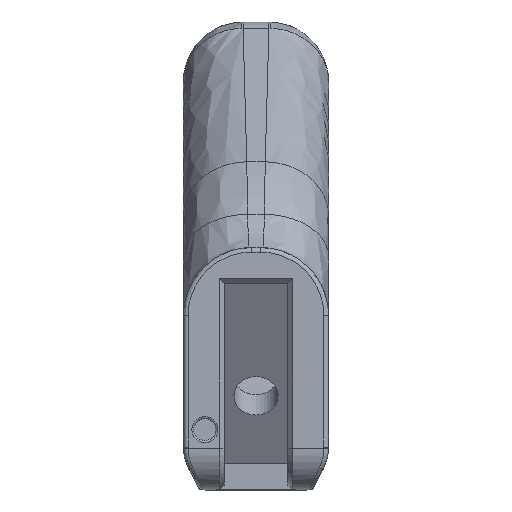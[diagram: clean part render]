
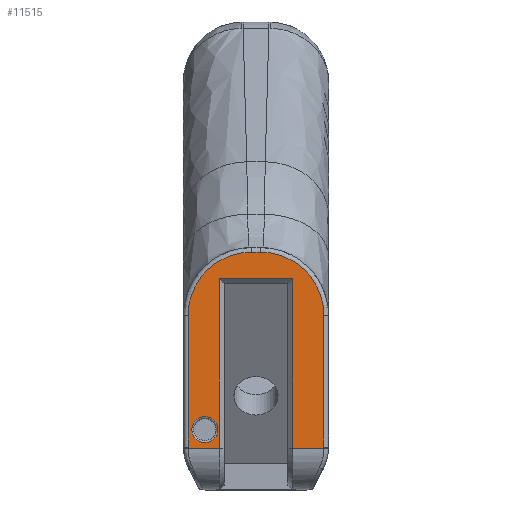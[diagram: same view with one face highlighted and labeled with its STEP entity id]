
A CAD part, top view. The second image highlights one B-rep face of the part: STEP entity #11515.
In plain terms, the highlighted planar face has unit normal (0, 0, 1).
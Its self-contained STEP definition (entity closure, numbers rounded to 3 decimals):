
#156=B_SPLINE_CURVE_WITH_KNOTS('',3,(#17221,#17222,#17223,#17224,#17225,
#17226),.UNSPECIFIED.,.F.,.F.,(4,1,1,4),(-0.785,-0.112,
0.337,0.785),.UNSPECIFIED.);
#157=B_SPLINE_CURVE_WITH_KNOTS('',3,(#17245,#17246,#17247,#17248,#17249,
#17250),.UNSPECIFIED.,.F.,.F.,(4,1,1,4),(-0.785,-0.112,
0.337,0.785),.UNSPECIFIED.);
#975=FACE_BOUND('',#3183,.T.);
#986=PLANE('',#12411);
#1139=LINE('',#17219,#1621);
#1140=LINE('',#17228,#1622);
#1141=LINE('',#17232,#1623);
#1142=LINE('',#17234,#1624);
#1143=LINE('',#17236,#1625);
#1144=LINE('',#17238,#1626);
#1145=LINE('',#17240,#1627);
#1146=LINE('',#17244,#1628);
#1621=VECTOR('',#13879,10.);
#1622=VECTOR('',#13880,10.);
#1623=VECTOR('',#13883,10.);
#1624=VECTOR('',#13884,10.);
#1625=VECTOR('',#13885,10.);
#1626=VECTOR('',#13886,10.);
#1627=VECTOR('',#13887,10.);
#1628=VECTOR('',#13890,10.);
#2375=FACE_OUTER_BOUND('',#3182,.T.);
#3182=EDGE_LOOP('',(#7882,#7883,#7884,#7885,#7886,#7887,#7888,#7889,#7890,
#7891,#7892,#7893));
#3183=EDGE_LOOP('',(#7894));
#4021=CIRCLE('',#12412,6.3);
#4022=CIRCLE('',#12413,6.3);
#4023=CIRCLE('',#12414,2.);
#4787=VERTEX_POINT('',#17217);
#4788=VERTEX_POINT('',#17218);
#4789=VERTEX_POINT('',#17220);
#4790=VERTEX_POINT('',#17227);
#4791=VERTEX_POINT('',#17229);
#4792=VERTEX_POINT('',#17231);
#4793=VERTEX_POINT('',#17233);
#4794=VERTEX_POINT('',#17235);
#4795=VERTEX_POINT('',#17237);
#4796=VERTEX_POINT('',#17239);
#4797=VERTEX_POINT('',#17241);
#4798=VERTEX_POINT('',#17243);
#4799=VERTEX_POINT('',#17251);
#5907=EDGE_CURVE('',#4787,#4788,#1139,.T.);
#5908=EDGE_CURVE('',#4789,#4787,#156,.T.);
#5909=EDGE_CURVE('',#4790,#4789,#1140,.T.);
#5910=EDGE_CURVE('',#4791,#4790,#4021,.T.);
#5911=EDGE_CURVE('',#4791,#4792,#1141,.T.);
#5912=EDGE_CURVE('',#4793,#4792,#1142,.T.);
#5913=EDGE_CURVE('',#4793,#4794,#1143,.T.);
#5914=EDGE_CURVE('',#4794,#4795,#1144,.T.);
#5915=EDGE_CURVE('',#4796,#4795,#1145,.T.);
#5916=EDGE_CURVE('',#4796,#4797,#4022,.T.);
#5917=EDGE_CURVE('',#4797,#4798,#1146,.T.);
#5918=EDGE_CURVE('',#4798,#4788,#157,.T.);
#5919=EDGE_CURVE('',#4799,#4799,#4023,.T.);
#7882=ORIENTED_EDGE('',*,*,#5907,.F.);
#7883=ORIENTED_EDGE('',*,*,#5908,.F.);
#7884=ORIENTED_EDGE('',*,*,#5909,.F.);
#7885=ORIENTED_EDGE('',*,*,#5910,.F.);
#7886=ORIENTED_EDGE('',*,*,#5911,.T.);
#7887=ORIENTED_EDGE('',*,*,#5912,.F.);
#7888=ORIENTED_EDGE('',*,*,#5913,.T.);
#7889=ORIENTED_EDGE('',*,*,#5914,.T.);
#7890=ORIENTED_EDGE('',*,*,#5915,.F.);
#7891=ORIENTED_EDGE('',*,*,#5916,.T.);
#7892=ORIENTED_EDGE('',*,*,#5917,.T.);
#7893=ORIENTED_EDGE('',*,*,#5918,.T.);
#7894=ORIENTED_EDGE('',*,*,#5919,.F.);
#11515=ADVANCED_FACE('',(#2375,#975),#986,.T.);
#12411=AXIS2_PLACEMENT_3D('',#17216,#13877,#13878);
#12412=AXIS2_PLACEMENT_3D('',#17230,#13881,#13882);
#12413=AXIS2_PLACEMENT_3D('',#17242,#13888,#13889);
#12414=AXIS2_PLACEMENT_3D('',#17252,#13891,#13892);
#13877=DIRECTION('center_axis',(0.,0.,
1.));
#13878=DIRECTION('ref_axis',(0.,-1.,0.));
#13879=DIRECTION('',(1.,0.,0.));
#13880=DIRECTION('',(0.,1.,0.));
#13881=DIRECTION('center_axis',(0.,0.,
-1.));
#13882=DIRECTION('ref_axis',(-1.,-0.015,0.));
#13883=DIRECTION('',(1.,0.,0.));
#13884=DIRECTION('',(0.,-1.,0.));
#13885=DIRECTION('',(1.,0.,0.));
#13886=DIRECTION('',(0.,-1.,0.));
#13887=DIRECTION('',(-1.,0.,0.));
#13888=DIRECTION('center_axis',(0.,0.,
1.));
#13889=DIRECTION('ref_axis',(1.,-0.015,0.));
#13890=DIRECTION('',(0.,1.,0.));
#13891=DIRECTION('center_axis',(0.,0.,
1.));
#13892=DIRECTION('ref_axis',(1.,0.,0.));
#17216=CARTESIAN_POINT('Origin',(19.207,-112.624,28.406));
#17217=CARTESIAN_POINT('',(23.407,-113.269,28.406));
#17218=CARTESIAN_POINT('',(24.756,-113.269,28.406));
#17219=CARTESIAN_POINT('',(27.226,-113.269,28.406));
#17220=CARTESIAN_POINT('',(13.618,-123.058,28.406));
#17221=CARTESIAN_POINT('Ctrl Pts',(13.618,-123.058,28.406));
#17222=CARTESIAN_POINT('Ctrl Pts',(13.618,-120.861,28.406));
#17223=CARTESIAN_POINT('Ctrl Pts',(14.902,-117.214,28.406));
#17224=CARTESIAN_POINT('Ctrl Pts',(19.019,-113.939,28.406));
#17225=CARTESIAN_POINT('Ctrl Pts',(21.943,-113.269,28.406));
#17226=CARTESIAN_POINT('Ctrl Pts',(23.407,-113.269,28.406));
#17227=CARTESIAN_POINT('',(13.618,-143.258,28.406));
#17228=CARTESIAN_POINT('',(13.618,-40.367,28.406));
#17229=CARTESIAN_POINT('',(13.622,-143.468,28.406));
#17230=CARTESIAN_POINT('Origin',(19.918,-143.258,28.406));
#17231=CARTESIAN_POINT('',(18.417,-143.468,28.406));
#17232=CARTESIAN_POINT('',(28.956,-143.468,28.406));
#17233=CARTESIAN_POINT('',(18.417,-117.318,28.406));
#17234=CARTESIAN_POINT('',(18.417,-114.618,28.406));
#17235=CARTESIAN_POINT('',(29.746,-117.318,28.406));
#17236=CARTESIAN_POINT('',(23.99,-117.318,28.406));
#17237=CARTESIAN_POINT('',(29.746,-143.468,28.406));
#17238=CARTESIAN_POINT('',(29.746,-114.618,28.406));
#17239=CARTESIAN_POINT('',(34.541,-143.468,28.406));
#17240=CARTESIAN_POINT('',(19.207,-143.468,28.406));
#17241=CARTESIAN_POINT('',(34.545,-143.258,28.406));
#17242=CARTESIAN_POINT('Origin',(28.245,-143.258,28.406));
#17243=CARTESIAN_POINT('',(34.545,-123.058,28.406));
#17244=CARTESIAN_POINT('',(34.545,-40.367,28.406));
#17245=CARTESIAN_POINT('Ctrl Pts',(34.545,-123.058,28.406));
#17246=CARTESIAN_POINT('Ctrl Pts',(34.545,-120.861,28.406));
#17247=CARTESIAN_POINT('Ctrl Pts',(33.261,-117.214,28.406));
#17248=CARTESIAN_POINT('Ctrl Pts',(29.144,-113.939,28.406));
#17249=CARTESIAN_POINT('Ctrl Pts',(26.22,-113.269,28.406));
#17250=CARTESIAN_POINT('Ctrl Pts',(24.756,-113.269,28.406));
#17251=CARTESIAN_POINT('',(18.205,-140.572,28.406));
#17252=CARTESIAN_POINT('Origin',(16.205,-140.572,28.406));
